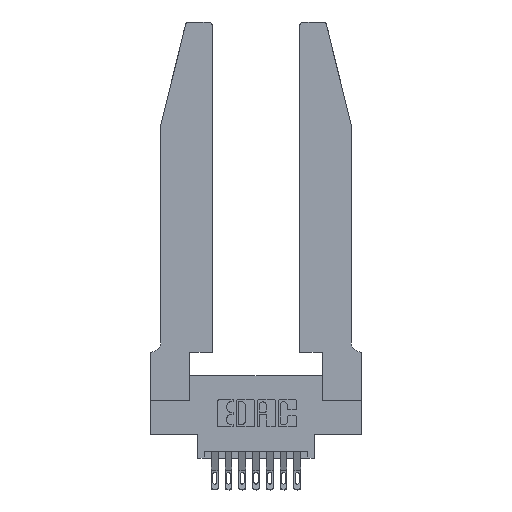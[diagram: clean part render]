
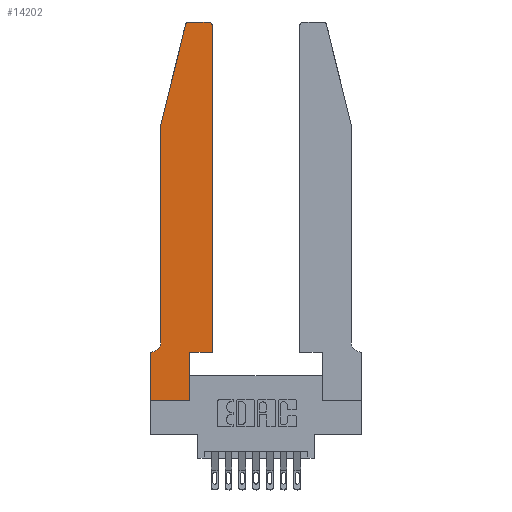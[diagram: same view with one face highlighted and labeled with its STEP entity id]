
A CAD part, top view. The second image highlights one B-rep face of the part: STEP entity #14202.
In plain terms, the highlighted planar face has unit normal (0, 0, 1).
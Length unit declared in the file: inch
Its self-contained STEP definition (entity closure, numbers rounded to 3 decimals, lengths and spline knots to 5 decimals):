
#389 = EDGE_CURVE ( 'NONE', #4364, #8709, #10948, .T. ) ;
#391 = DIRECTION ( 'NONE',  ( 0., 0., 1. ) ) ;
#579 = ORIENTED_EDGE ( 'NONE', *, *, #7193, .T. ) ;
#722 = DIRECTION ( 'NONE',  ( -0.239, -0.971, 0. ) ) ;
#773 = VERTEX_POINT ( 'NONE', #1192 ) ;
#834 = CARTESIAN_POINT ( 'NONE',  ( 0.4205, 2.75, 0.37 ) ) ;
#850 = CARTESIAN_POINT ( 'NONE',  ( 0.284, 2.75, 0.37 ) ) ;
#901 = VECTOR ( 'NONE', #8060, 39.37008 ) ;
#1116 = AXIS2_PLACEMENT_3D ( 'NONE', #14348, #10921, #1442 ) ;
#1123 = CARTESIAN_POINT ( 'NONE',  ( 0.4505, 0.35, 0.37 ) ) ;
#1192 = CARTESIAN_POINT ( 'NONE',  ( 0.0755, 2., 0.37 ) ) ;
#1340 = VERTEX_POINT ( 'NONE', #9823 ) ;
#1442 = DIRECTION ( 'NONE',  ( -1., 0., 0. ) ) ;
#1498 = ORIENTED_EDGE ( 'NONE', *, *, #3967, .T. ) ;
#1502 = VECTOR ( 'NONE', #6153, 39.37008 ) ;
#1662 = DIRECTION ( 'NONE',  ( -1., 0., 0. ) ) ;
#1699 = CARTESIAN_POINT ( 'NONE',  ( 0., 0.35, 0.37 ) ) ;
#1703 = CARTESIAN_POINT ( 'NONE',  ( 0.4205, 2.72, 0.37 ) ) ;
#1791 = DIRECTION ( 'NONE',  ( 0., 1., 0. ) ) ;
#1853 = CARTESIAN_POINT ( 'NONE',  ( 0., 0., 0.37 ) ) ;
#1878 = CARTESIAN_POINT ( 'NONE',  ( 0.0755, 2., 0.37 ) ) ;
#2151 = VECTOR ( 'NONE', #1791, 39.37008 ) ;
#2244 = ORIENTED_EDGE ( 'NONE', *, *, #6867, .T. ) ;
#2331 = ORIENTED_EDGE ( 'NONE', *, *, #12486, .T. ) ;
#2348 = VERTEX_POINT ( 'NONE', #834 ) ;
#2573 = AXIS2_PLACEMENT_3D ( 'NONE', #1703, #6553, #5219 ) ;
#2618 = ORIENTED_EDGE ( 'NONE', *, *, #7876, .T. ) ;
#2641 = EDGE_CURVE ( 'NONE', #13961, #2348, #6295, .T. ) ;
#2757 = LINE ( 'NONE', #15243, #901 ) ;
#2844 = FACE_OUTER_BOUND ( 'NONE', #3374, .T. ) ;
#3224 = ORIENTED_EDGE ( 'NONE', *, *, #389, .T. ) ;
#3282 = EDGE_CURVE ( 'NONE', #6136, #13116, #6957, .T. ) ;
#3315 = VECTOR ( 'NONE', #4233, 39.37008 ) ;
#3374 = EDGE_LOOP ( 'NONE', ( #7125, #8874, #6510, #2244, #579, #2331, #1498, #3224, #9688, #2618, #13938, #8372 ) ) ;
#3736 = VERTEX_POINT ( 'NONE', #1699 ) ;
#3932 = DIRECTION ( 'NONE',  ( 1., 0., 0. ) ) ;
#3967 = EDGE_CURVE ( 'NONE', #3736, #4364, #10527, .T. ) ;
#4233 = DIRECTION ( 'NONE',  ( 1., 0., 0. ) ) ;
#4364 = VERTEX_POINT ( 'NONE', #1853 ) ;
#4843 = CARTESIAN_POINT ( 'NONE',  ( 0.0055, 0.35, 0.37 ) ) ;
#5004 = CARTESIAN_POINT ( 'NONE',  ( 0.2865, 0.35, 0.37 ) ) ;
#5055 = CARTESIAN_POINT ( 'NONE',  ( 0.0755, 0.35, 0.37 ) ) ;
#5219 = DIRECTION ( 'NONE',  ( 1., 0., 0. ) ) ;
#5611 = LINE ( 'NONE', #7455, #12488 ) ;
#6136 = VERTEX_POINT ( 'NONE', #850 ) ;
#6153 = DIRECTION ( 'NONE',  ( 1., 0., 0. ) ) ;
#6244 = DIRECTION ( 'NONE',  ( -1., 0., 0. ) ) ;
#6295 = CIRCLE ( 'NONE', #2573, 0.03 ) ;
#6459 = CARTESIAN_POINT ( 'NONE',  ( 0.284, 2.72, 0.37 ) ) ;
#6510 = ORIENTED_EDGE ( 'NONE', *, *, #15006, .T. ) ;
#6553 = DIRECTION ( 'NONE',  ( 0., 0., 1. ) ) ;
#6867 = EDGE_CURVE ( 'NONE', #773, #10714, #13360, .T. ) ;
#6918 = LINE ( 'NONE', #8674, #2151 ) ;
#6957 = CIRCLE ( 'NONE', #13596, 0.03 ) ;
#7125 = ORIENTED_EDGE ( 'NONE', *, *, #14861, .T. ) ;
#7193 = EDGE_CURVE ( 'NONE', #10714, #9428, #8311, .T. ) ;
#7455 = CARTESIAN_POINT ( 'NONE',  ( 0.2605, 2.75, 0.37 ) ) ;
#7565 = EDGE_CURVE ( 'NONE', #1340, #13961, #2757, .T. ) ;
#7763 = DIRECTION ( 'NONE',  ( 0., -1., 0. ) ) ;
#7828 = AXIS2_PLACEMENT_3D ( 'NONE', #12307, #11044, #3932 ) ;
#7876 = EDGE_CURVE ( 'NONE', #10816, #1340, #14290, .T. ) ;
#7912 = CARTESIAN_POINT ( 'NONE',  ( 0.0755, 2., 0.37 ) ) ;
#8060 = DIRECTION ( 'NONE',  ( 0., 1., 0. ) ) ;
#8184 = VECTOR ( 'NONE', #722, 39.37008 ) ;
#8311 = CIRCLE ( 'NONE', #1116, 0.07 ) ;
#8372 = ORIENTED_EDGE ( 'NONE', *, *, #2641, .T. ) ;
#8423 = CARTESIAN_POINT ( 'NONE',  ( 0.0755, 0.42, 0.37 ) ) ;
#8674 = CARTESIAN_POINT ( 'NONE',  ( 0.2865, 0.35, 0.37 ) ) ;
#8709 = VERTEX_POINT ( 'NONE', #9405 ) ;
#8874 = ORIENTED_EDGE ( 'NONE', *, *, #3282, .T. ) ;
#9237 = VECTOR ( 'NONE', #7763, 39.37008 ) ;
#9405 = CARTESIAN_POINT ( 'NONE',  ( 0.2865, 0., 0.37 ) ) ;
#9428 = VERTEX_POINT ( 'NONE', #4843 ) ;
#9688 = ORIENTED_EDGE ( 'NONE', *, *, #11354, .T. ) ;
#9823 = CARTESIAN_POINT ( 'NONE',  ( 0.4505, 0.35, 0.37 ) ) ;
#10527 = LINE ( 'NONE', #10944, #12197 ) ;
#10714 = VERTEX_POINT ( 'NONE', #8423 ) ;
#10816 = VERTEX_POINT ( 'NONE', #5004 ) ;
#10921 = DIRECTION ( 'NONE',  ( 0., 0., -1. ) ) ;
#10926 = CARTESIAN_POINT ( 'NONE',  ( 0., 0., 0.37 ) ) ;
#10944 = CARTESIAN_POINT ( 'NONE',  ( 0., 0., 0.37 ) ) ;
#10948 = LINE ( 'NONE', #10926, #1502 ) ;
#11044 = DIRECTION ( 'NONE',  ( 0., 0., 1. ) ) ;
#11354 = EDGE_CURVE ( 'NONE', #8709, #10816, #6918, .T. ) ;
#12103 = LINE ( 'NONE', #7912, #8184 ) ;
#12197 = VECTOR ( 'NONE', #12204, 39.37008 ) ;
#12204 = DIRECTION ( 'NONE',  ( 0., -1., 0. ) ) ;
#12307 = CARTESIAN_POINT ( 'NONE',  ( 0., 0.35, 0.37 ) ) ;
#12420 = CARTESIAN_POINT ( 'NONE',  ( 0.25487, 2.72718, 0.37 ) ) ;
#12486 = EDGE_CURVE ( 'NONE', #9428, #3736, #15207, .T. ) ;
#12488 = VECTOR ( 'NONE', #1662, 39.37008 ) ;
#12556 = VECTOR ( 'NONE', #6244, 39.37008 ) ;
#13005 = CARTESIAN_POINT ( 'NONE',  ( 0.4505, 2.72, 0.37 ) ) ;
#13116 = VERTEX_POINT ( 'NONE', #12420 ) ;
#13360 = LINE ( 'NONE', #1878, #9237 ) ;
#13543 = PLANE ( 'NONE',  #7828 ) ;
#13596 = AXIS2_PLACEMENT_3D ( 'NONE', #6459, #391, #14712 ) ;
#13938 = ORIENTED_EDGE ( 'NONE', *, *, #7565, .T. ) ;
#13961 = VERTEX_POINT ( 'NONE', #13005 ) ;
#14202 = ADVANCED_FACE ( 'NONE', ( #2844 ), #13543, .T. ) ;
#14290 = LINE ( 'NONE', #1123, #3315 ) ;
#14348 = CARTESIAN_POINT ( 'NONE',  ( 0.0055, 0.42, 0.37 ) ) ;
#14712 = DIRECTION ( 'NONE',  ( 1., 0., 0. ) ) ;
#14861 = EDGE_CURVE ( 'NONE', #2348, #6136, #5611, .T. ) ;
#15006 = EDGE_CURVE ( 'NONE', #13116, #773, #12103, .T. ) ;
#15207 = LINE ( 'NONE', #5055, #12556 ) ;
#15243 = CARTESIAN_POINT ( 'NONE',  ( 0.4505, 0.35, 0.37 ) ) ;
